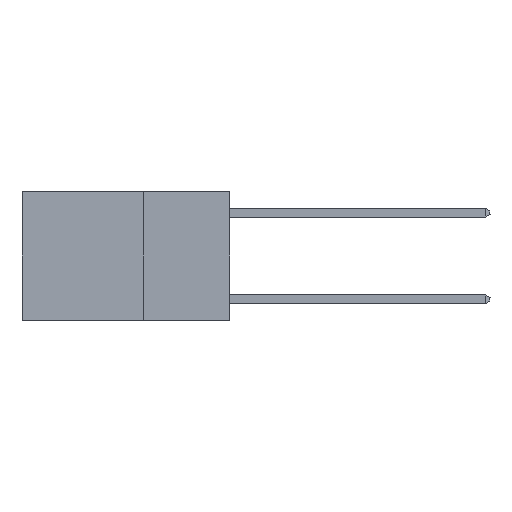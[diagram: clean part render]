
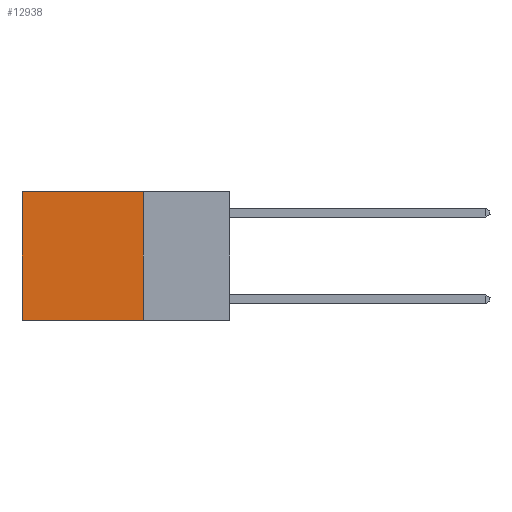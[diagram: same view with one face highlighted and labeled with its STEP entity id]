
A CAD part, left-side view. The second image highlights one B-rep face of the part: STEP entity #12938.
In plain terms, the highlighted planar face has unit normal (-1, 0, 0).
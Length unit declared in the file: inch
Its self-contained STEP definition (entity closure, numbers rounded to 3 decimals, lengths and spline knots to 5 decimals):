
#903 = CARTESIAN_POINT ( 'NONE',  ( 0.2625, 0.6, -0.37 ) ) ;
#2699 = VECTOR ( 'NONE', #21237, 39.37008 ) ;
#2795 = ORIENTED_EDGE ( 'NONE', *, *, #20715, .F. ) ;
#3201 = DIRECTION ( 'NONE',  ( 0., 0., -1. ) ) ;
#4005 = CARTESIAN_POINT ( 'NONE',  ( 0.2625, 0.6, 0. ) ) ;
#4334 = EDGE_CURVE ( 'NONE', #14789, #16813, #4821, .T. ) ;
#4821 = LINE ( 'NONE', #23859, #10737 ) ;
#4932 = CARTESIAN_POINT ( 'NONE',  ( 0.2625, 0.25, 0. ) ) ;
#5876 = LINE ( 'NONE', #4005, #23875 ) ;
#6153 = ORIENTED_EDGE ( 'NONE', *, *, #13298, .F. ) ;
#6262 = EDGE_LOOP ( 'NONE', ( #15620, #6153, #2795, #13931 ) ) ;
#6665 = DIRECTION ( 'NONE',  ( 1., 0., 0. ) ) ;
#10457 = PLANE ( 'NONE',  #19154 ) ;
#10737 = VECTOR ( 'NONE', #22133, 39.37008 ) ;
#10994 = EDGE_CURVE ( 'NONE', #16813, #22613, #5876, .T. ) ;
#12938 = ADVANCED_FACE ( 'NONE', ( #17835 ), #10457, .F. ) ;
#13079 = VECTOR ( 'NONE', #18018, 39.37008 ) ;
#13298 = EDGE_CURVE ( 'NONE', #18986, #22613, #13392, .T. ) ;
#13392 = LINE ( 'NONE', #20872, #2699 ) ;
#13931 = ORIENTED_EDGE ( 'NONE', *, *, #4334, .T. ) ;
#14789 = VERTEX_POINT ( 'NONE', #20003 ) ;
#15620 = ORIENTED_EDGE ( 'NONE', *, *, #10994, .T. ) ;
#16530 = CARTESIAN_POINT ( 'NONE',  ( 0.2625, 0.6, 0. ) ) ;
#16813 = VERTEX_POINT ( 'NONE', #16530 ) ;
#17835 = FACE_OUTER_BOUND ( 'NONE', #6262, .T. ) ;
#18018 = DIRECTION ( 'NONE',  ( 0., 0., -1. ) ) ;
#18986 = VERTEX_POINT ( 'NONE', #20398 ) ;
#19123 = DIRECTION ( 'NONE',  ( 0., 0., -1. ) ) ;
#19154 = AXIS2_PLACEMENT_3D ( 'NONE', #4932, #6665, #3201 ) ;
#19720 = LINE ( 'NONE', #19836, #13079 ) ;
#19836 = CARTESIAN_POINT ( 'NONE',  ( 0.2625, 0.25, 0. ) ) ;
#20003 = CARTESIAN_POINT ( 'NONE',  ( 0.2625, 0.25, 0. ) ) ;
#20398 = CARTESIAN_POINT ( 'NONE',  ( 0.2625, 0.25, -0.37 ) ) ;
#20715 = EDGE_CURVE ( 'NONE', #14789, #18986, #19720, .T. ) ;
#20872 = CARTESIAN_POINT ( 'NONE',  ( 0.2625, 0.25, -0.37 ) ) ;
#21237 = DIRECTION ( 'NONE',  ( 0., 1., 0. ) ) ;
#22133 = DIRECTION ( 'NONE',  ( 0., 1., 0. ) ) ;
#22613 = VERTEX_POINT ( 'NONE', #903 ) ;
#23859 = CARTESIAN_POINT ( 'NONE',  ( 0.2625, 0.25, 0. ) ) ;
#23875 = VECTOR ( 'NONE', #19123, 39.37008 ) ;
